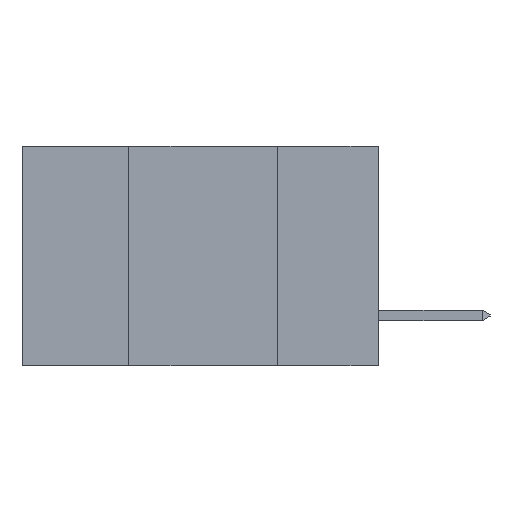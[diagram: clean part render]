
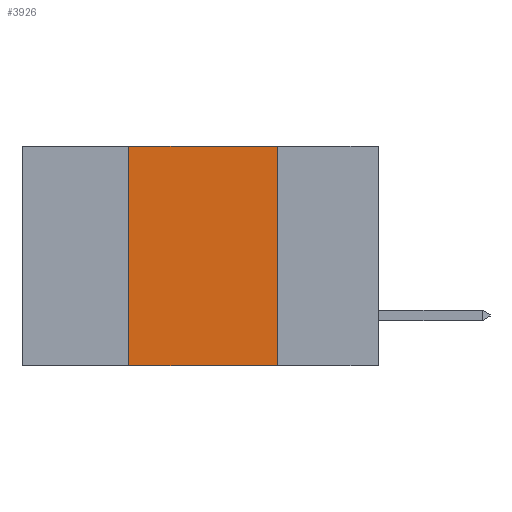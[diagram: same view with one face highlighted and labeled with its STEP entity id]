
A CAD part, left-side view. The second image highlights one B-rep face of the part: STEP entity #3926.
In plain terms, the highlighted planar face has unit normal (-1, 0, 0).
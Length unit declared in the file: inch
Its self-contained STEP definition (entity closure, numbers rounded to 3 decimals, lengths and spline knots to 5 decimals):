
#163 = EDGE_CURVE ( 'NONE', #1970, #2093, #1120, .T. ) ;
#184 = DIRECTION ( 'NONE',  ( 0., 0., -1. ) ) ;
#216 = DIRECTION ( 'NONE',  ( 1., 0., 0. ) ) ;
#322 = VERTEX_POINT ( 'NONE', #1549 ) ;
#621 = ORIENTED_EDGE ( 'NONE', *, *, #163, .F. ) ;
#747 = LINE ( 'NONE', #8093, #6299 ) ;
#1120 = LINE ( 'NONE', #5538, #3660 ) ;
#1549 = CARTESIAN_POINT ( 'NONE',  ( 0., 0.42, -0.37 ) ) ;
#1583 = DIRECTION ( 'NONE',  ( 0., 0., 1. ) ) ;
#1970 = VERTEX_POINT ( 'NONE', #7732 ) ;
#2093 = VERTEX_POINT ( 'NONE', #2684 ) ;
#2431 = EDGE_LOOP ( 'NONE', ( #6642, #621, #4449, #8069 ) ) ;
#2684 = CARTESIAN_POINT ( 'NONE',  ( 0., 0.17, 0. ) ) ;
#3204 = LINE ( 'NONE', #9547, #8741 ) ;
#3660 = VECTOR ( 'NONE', #6568, 39.37008 ) ;
#3926 = ADVANCED_FACE ( 'NONE', ( #6146 ), #4604, .F. ) ;
#4449 = ORIENTED_EDGE ( 'NONE', *, *, #8635, .F. ) ;
#4604 = PLANE ( 'NONE',  #9202 ) ;
#4729 = CARTESIAN_POINT ( 'NONE',  ( 0., 0.6, 0. ) ) ;
#5301 = EDGE_CURVE ( 'NONE', #2093, #7234, #747, .T. ) ;
#5362 = EDGE_CURVE ( 'NONE', #322, #7234, #6084, .T. ) ;
#5538 = CARTESIAN_POINT ( 'NONE',  ( 0., 0.6, 0. ) ) ;
#6084 = LINE ( 'NONE', #8672, #9532 ) ;
#6146 = FACE_OUTER_BOUND ( 'NONE', #2431, .T. ) ;
#6299 = VECTOR ( 'NONE', #7933, 39.37008 ) ;
#6568 = DIRECTION ( 'NONE',  ( 0., -1., 0. ) ) ;
#6642 = ORIENTED_EDGE ( 'NONE', *, *, #5301, .F. ) ;
#7234 = VERTEX_POINT ( 'NONE', #8702 ) ;
#7732 = CARTESIAN_POINT ( 'NONE',  ( 0., 0.42, 0. ) ) ;
#7933 = DIRECTION ( 'NONE',  ( 0., 0., -1. ) ) ;
#8069 = ORIENTED_EDGE ( 'NONE', *, *, #5362, .T. ) ;
#8093 = CARTESIAN_POINT ( 'NONE',  ( 0., 0.17, -0.37 ) ) ;
#8551 = DIRECTION ( 'NONE',  ( 0., -1., 0. ) ) ;
#8635 = EDGE_CURVE ( 'NONE', #322, #1970, #3204, .T. ) ;
#8672 = CARTESIAN_POINT ( 'NONE',  ( 0., 0.6, -0.37 ) ) ;
#8702 = CARTESIAN_POINT ( 'NONE',  ( 0., 0.17, -0.37 ) ) ;
#8741 = VECTOR ( 'NONE', #1583, 39.37008 ) ;
#9202 = AXIS2_PLACEMENT_3D ( 'NONE', #4729, #216, #184 ) ;
#9532 = VECTOR ( 'NONE', #8551, 39.37008 ) ;
#9547 = CARTESIAN_POINT ( 'NONE',  ( 0., 0.42, -0.37 ) ) ;
